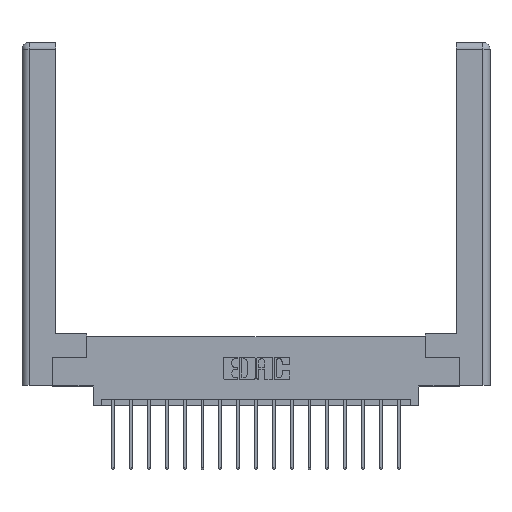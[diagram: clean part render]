
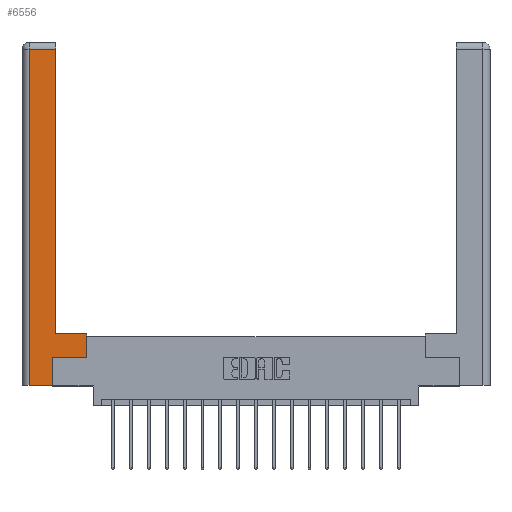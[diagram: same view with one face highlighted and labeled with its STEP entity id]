
A CAD part, top view. The second image highlights one B-rep face of the part: STEP entity #6556.
In plain terms, the highlighted planar face has unit normal (0, 0, 1).
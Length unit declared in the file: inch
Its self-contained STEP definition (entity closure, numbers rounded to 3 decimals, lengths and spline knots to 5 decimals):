
#144 = ORIENTED_EDGE ( 'NONE', *, *, #17680, .T. ) ;
#365 = VERTEX_POINT ( 'NONE', #15796 ) ;
#745 = DIRECTION ( 'NONE',  ( 0., 1., 0. ) ) ;
#810 = CARTESIAN_POINT ( 'NONE',  ( 0.265, 0., 0. ) ) ;
#876 = EDGE_CURVE ( 'NONE', #365, #11624, #2353, .T. ) ;
#968 = VECTOR ( 'NONE', #4409, 39.37008 ) ;
#1253 = AXIS2_PLACEMENT_3D ( 'NONE', #11014, #15502, #13984 ) ;
#1631 = LINE ( 'NONE', #14902, #16021 ) ;
#1884 = CARTESIAN_POINT ( 'NONE',  ( 0.565, 0.45, 0. ) ) ;
#2062 = ORIENTED_EDGE ( 'NONE', *, *, #14541, .T. ) ;
#2353 = LINE ( 'NONE', #10370, #968 ) ;
#2440 = CARTESIAN_POINT ( 'NONE',  ( 0.565, 0.245, 0. ) ) ;
#2873 = CARTESIAN_POINT ( 'NONE',  ( 0.0615, 2.94, 0. ) ) ;
#2881 = LINE ( 'NONE', #11570, #5609 ) ;
#3074 = VERTEX_POINT ( 'NONE', #13427 ) ;
#3231 = DIRECTION ( 'NONE',  ( 0., -1., 0. ) ) ;
#3362 = CARTESIAN_POINT ( 'NONE',  ( 0.0615, 0., 0. ) ) ;
#4400 = VERTEX_POINT ( 'NONE', #810 ) ;
#4409 = DIRECTION ( 'NONE',  ( -1., 0., 0. ) ) ;
#5609 = VECTOR ( 'NONE', #7055, 39.37008 ) ;
#6504 = DIRECTION ( 'NONE',  ( -1., 0., 0. ) ) ;
#6556 = ADVANCED_FACE ( 'NONE', ( #13277 ), #16965, .F. ) ;
#6617 = ORIENTED_EDGE ( 'NONE', *, *, #876, .T. ) ;
#7055 = DIRECTION ( 'NONE',  ( 1., 0., 0. ) ) ;
#7289 = ORIENTED_EDGE ( 'NONE', *, *, #8788, .T. ) ;
#8216 = CARTESIAN_POINT ( 'NONE',  ( 0.295, 0.45, 0. ) ) ;
#8667 = DIRECTION ( 'NONE',  ( 1., 0., 0. ) ) ;
#8788 = EDGE_CURVE ( 'NONE', #3074, #9838, #2881, .T. ) ;
#9060 = LINE ( 'NONE', #13818, #14882 ) ;
#9444 = EDGE_CURVE ( 'NONE', #12108, #365, #18694, .T. ) ;
#9838 = VERTEX_POINT ( 'NONE', #2440 ) ;
#10159 = CARTESIAN_POINT ( 'NONE',  ( 0.0615, 0., 0. ) ) ;
#10370 = CARTESIAN_POINT ( 'NONE',  ( 0.0615, 2.94, 0. ) ) ;
#10550 = ORIENTED_EDGE ( 'NONE', *, *, #9444, .T. ) ;
#11014 = CARTESIAN_POINT ( 'NONE',  ( 0., 0., 0. ) ) ;
#11146 = VECTOR ( 'NONE', #12388, 39.37008 ) ;
#11325 = EDGE_LOOP ( 'NONE', ( #10550, #6617, #13939, #2062, #18433, #7289, #144, #12769 ) ) ;
#11570 = CARTESIAN_POINT ( 'NONE',  ( 0.565, 0.245, 0. ) ) ;
#11624 = VERTEX_POINT ( 'NONE', #2873 ) ;
#11629 = EDGE_CURVE ( 'NONE', #4400, #3074, #1631, .T. ) ;
#12086 = CARTESIAN_POINT ( 'NONE',  ( 0.565, 0.45, 0. ) ) ;
#12108 = VERTEX_POINT ( 'NONE', #8216 ) ;
#12388 = DIRECTION ( 'NONE',  ( 0., 1., 0. ) ) ;
#12769 = ORIENTED_EDGE ( 'NONE', *, *, #16365, .T. ) ;
#13263 = CARTESIAN_POINT ( 'NONE',  ( 0.265, 0., 0. ) ) ;
#13277 = FACE_OUTER_BOUND ( 'NONE', #11325, .T. ) ;
#13427 = CARTESIAN_POINT ( 'NONE',  ( 0.265, 0.245, 0. ) ) ;
#13818 = CARTESIAN_POINT ( 'NONE',  ( 0.295, 0.45, 0. ) ) ;
#13939 = ORIENTED_EDGE ( 'NONE', *, *, #17939, .T. ) ;
#13984 = DIRECTION ( 'NONE',  ( -1., 0., 0. ) ) ;
#14014 = VECTOR ( 'NONE', #8667, 39.37008 ) ;
#14541 = EDGE_CURVE ( 'NONE', #16750, #4400, #16557, .T. ) ;
#14882 = VECTOR ( 'NONE', #6504, 39.37008 ) ;
#14902 = CARTESIAN_POINT ( 'NONE',  ( 0.265, 0.245, 0. ) ) ;
#15502 = DIRECTION ( 'NONE',  ( 0., 0., -1. ) ) ;
#15796 = CARTESIAN_POINT ( 'NONE',  ( 0.295, 2.94, 0. ) ) ;
#16005 = LINE ( 'NONE', #1884, #11146 ) ;
#16021 = VECTOR ( 'NONE', #16381, 39.37008 ) ;
#16365 = EDGE_CURVE ( 'NONE', #19200, #12108, #9060, .T. ) ;
#16381 = DIRECTION ( 'NONE',  ( 0., 1., 0. ) ) ;
#16557 = LINE ( 'NONE', #13263, #14014 ) ;
#16750 = VERTEX_POINT ( 'NONE', #10159 ) ;
#16965 = PLANE ( 'NONE',  #1253 ) ;
#17086 = CARTESIAN_POINT ( 'NONE',  ( 0.295, 3., 0. ) ) ;
#17680 = EDGE_CURVE ( 'NONE', #9838, #19200, #16005, .T. ) ;
#17939 = EDGE_CURVE ( 'NONE', #11624, #16750, #19012, .T. ) ;
#18089 = VECTOR ( 'NONE', #3231, 39.37008 ) ;
#18433 = ORIENTED_EDGE ( 'NONE', *, *, #11629, .T. ) ;
#18694 = LINE ( 'NONE', #17086, #18912 ) ;
#18912 = VECTOR ( 'NONE', #745, 39.37008 ) ;
#19012 = LINE ( 'NONE', #3362, #18089 ) ;
#19200 = VERTEX_POINT ( 'NONE', #12086 ) ;
